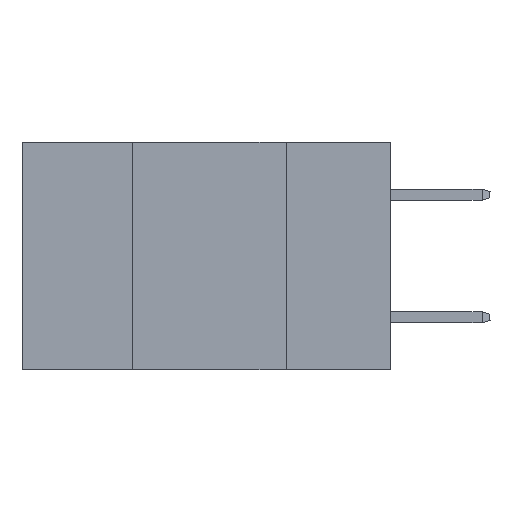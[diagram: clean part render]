
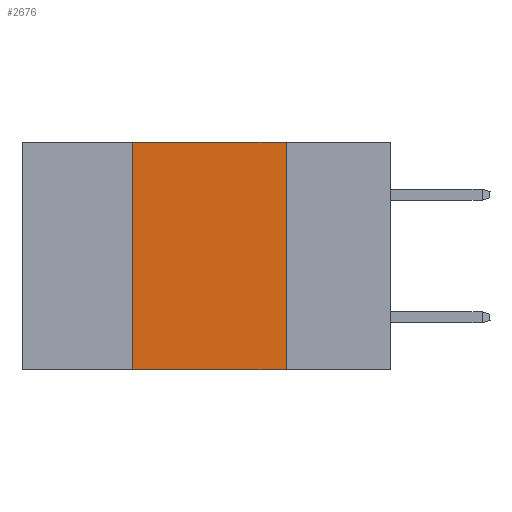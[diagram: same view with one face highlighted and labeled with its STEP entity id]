
A CAD part, left-side view. The second image highlights one B-rep face of the part: STEP entity #2676.
In plain terms, the highlighted planar face has unit normal (-1, 0, 0).
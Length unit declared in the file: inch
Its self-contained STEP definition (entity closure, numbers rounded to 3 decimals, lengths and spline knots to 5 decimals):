
#313 = VERTEX_POINT ( 'NONE', #2452 ) ;
#1462 = DIRECTION ( 'NONE',  ( 1., 0., 0. ) ) ;
#1552 = EDGE_CURVE ( 'NONE', #3387, #6700, #14111, .T. ) ;
#1777 = EDGE_CURVE ( 'NONE', #3387, #313, #15033, .T. ) ;
#2257 = VERTEX_POINT ( 'NONE', #11237 ) ;
#2452 = CARTESIAN_POINT ( 'NONE',  ( 0., 0.17, -0.37 ) ) ;
#2676 = ADVANCED_FACE ( 'NONE', ( #12599 ), #2782, .F. ) ;
#2782 = PLANE ( 'NONE',  #8544 ) ;
#3037 = DIRECTION ( 'NONE',  ( 0., -1., 0. ) ) ;
#3355 = CARTESIAN_POINT ( 'NONE',  ( 0., 0.42, 0. ) ) ;
#3387 = VERTEX_POINT ( 'NONE', #8639 ) ;
#3955 = CARTESIAN_POINT ( 'NONE',  ( 0., 0.17, 0. ) ) ;
#5134 = DIRECTION ( 'NONE',  ( 0., -1., 0. ) ) ;
#5565 = ORIENTED_EDGE ( 'NONE', *, *, #1552, .F. ) ;
#5783 = EDGE_CURVE ( 'NONE', #6700, #2257, #15808, .T. ) ;
#5856 = CARTESIAN_POINT ( 'NONE',  ( 0., 0.6, 0. ) ) ;
#5897 = ORIENTED_EDGE ( 'NONE', *, *, #5783, .F. ) ;
#6295 = EDGE_LOOP ( 'NONE', ( #12150, #5897, #5565, #13306 ) ) ;
#6502 = DIRECTION ( 'NONE',  ( 0., 0., 1. ) ) ;
#6700 = VERTEX_POINT ( 'NONE', #9585 ) ;
#7807 = VECTOR ( 'NONE', #6502, 39.37008 ) ;
#8281 = DIRECTION ( 'NONE',  ( 0., 0., -1. ) ) ;
#8544 = AXIS2_PLACEMENT_3D ( 'NONE', #10626, #1462, #8281 ) ;
#8639 = CARTESIAN_POINT ( 'NONE',  ( 0., 0.42, -0.37 ) ) ;
#8692 = LINE ( 'NONE', #3955, #13862 ) ;
#9282 = CARTESIAN_POINT ( 'NONE',  ( 0., 0.6, -0.37 ) ) ;
#9585 = CARTESIAN_POINT ( 'NONE',  ( 0., 0.42, 0. ) ) ;
#10626 = CARTESIAN_POINT ( 'NONE',  ( 0., 0.6, 0. ) ) ;
#11237 = CARTESIAN_POINT ( 'NONE',  ( 0., 0.17, 0. ) ) ;
#11499 = VECTOR ( 'NONE', #3037, 39.37008 ) ;
#12150 = ORIENTED_EDGE ( 'NONE', *, *, #12505, .F. ) ;
#12505 = EDGE_CURVE ( 'NONE', #2257, #313, #8692, .T. ) ;
#12599 = FACE_OUTER_BOUND ( 'NONE', #6295, .T. ) ;
#13306 = ORIENTED_EDGE ( 'NONE', *, *, #1777, .T. ) ;
#13862 = VECTOR ( 'NONE', #14903, 39.37008 ) ;
#14111 = LINE ( 'NONE', #3355, #7807 ) ;
#14903 = DIRECTION ( 'NONE',  ( 0., 0., -1. ) ) ;
#15033 = LINE ( 'NONE', #9282, #11499 ) ;
#15445 = VECTOR ( 'NONE', #5134, 39.37008 ) ;
#15808 = LINE ( 'NONE', #5856, #15445 ) ;
